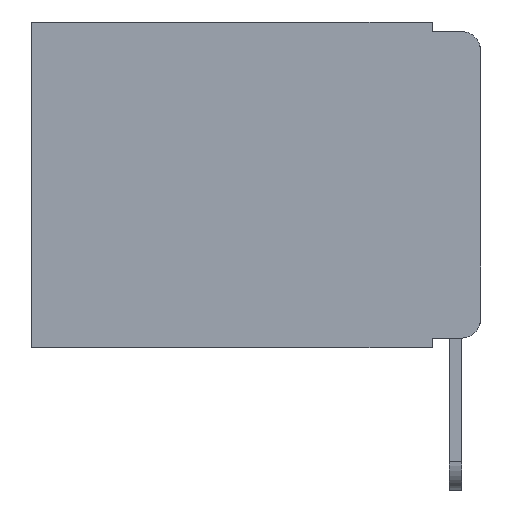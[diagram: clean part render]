
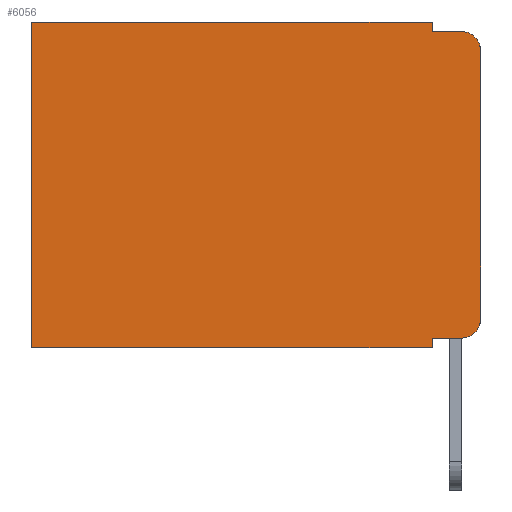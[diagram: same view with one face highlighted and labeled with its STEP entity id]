
A CAD part, left-side view. The second image highlights one B-rep face of the part: STEP entity #6056.
In plain terms, the highlighted planar face has unit normal (-1, 0, 0).
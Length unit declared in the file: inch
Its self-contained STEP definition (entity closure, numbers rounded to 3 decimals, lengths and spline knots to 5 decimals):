
#181 = CARTESIAN_POINT ( 'NONE',  ( 0.298, 0.051, -0.333 ) ) ;
#778 = PLANE ( 'NONE',  #12968 ) ;
#1369 = EDGE_CURVE ( 'NONE', #5572, #11298, #10958, .T. ) ;
#1847 = VECTOR ( 'NONE', #14663, 39.37008 ) ;
#2580 = CARTESIAN_POINT ( 'NONE',  ( 0.298, 0.02, -0.03 ) ) ;
#3357 = LINE ( 'NONE', #17226, #19488 ) ;
#3425 = DIRECTION ( 'NONE',  ( 0., 0., -1. ) ) ;
#3515 = CARTESIAN_POINT ( 'NONE',  ( 0.298, 0., -0.343 ) ) ;
#3864 = CARTESIAN_POINT ( 'NONE',  ( 0.298, 0.473, 0. ) ) ;
#4097 = EDGE_CURVE ( 'NONE', #12033, #11298, #12627, .T. ) ;
#4200 = DIRECTION ( 'NONE',  ( 0., 0., -1. ) ) ;
#4213 = EDGE_CURVE ( 'NONE', #16299, #5541, #19258, .T. ) ;
#4324 = VECTOR ( 'NONE', #3425, 39.37008 ) ;
#4493 = EDGE_CURVE ( 'NONE', #6920, #5959, #15123, .T. ) ;
#4494 = ORIENTED_EDGE ( 'NONE', *, *, #1369, .F. ) ;
#4986 = VERTEX_POINT ( 'NONE', #16802 ) ;
#5541 = VERTEX_POINT ( 'NONE', #6216 ) ;
#5571 = VECTOR ( 'NONE', #18722, 39.37008 ) ;
#5572 = VERTEX_POINT ( 'NONE', #7860 ) ;
#5959 = VERTEX_POINT ( 'NONE', #6481 ) ;
#6010 = EDGE_CURVE ( 'NONE', #5959, #4986, #3357, .T. ) ;
#6024 = ORIENTED_EDGE ( 'NONE', *, *, #19895, .T. ) ;
#6056 = ADVANCED_FACE ( 'NONE', ( #15126 ), #778, .F. ) ;
#6216 = CARTESIAN_POINT ( 'NONE',  ( 0.298, 0., -0.313 ) ) ;
#6302 = EDGE_CURVE ( 'NONE', #15396, #5572, #16956, .T. ) ;
#6419 = CARTESIAN_POINT ( 'NONE',  ( 0.298, 0.473, 0. ) ) ;
#6420 = VECTOR ( 'NONE', #18588, 39.37008 ) ;
#6481 = CARTESIAN_POINT ( 'NONE',  ( 0.298, 0.051, -0.01 ) ) ;
#6900 = CARTESIAN_POINT ( 'NONE',  ( 0.298, 0., -0.03 ) ) ;
#6920 = VERTEX_POINT ( 'NONE', #14558 ) ;
#7513 = ORIENTED_EDGE ( 'NONE', *, *, #9626, .T. ) ;
#7668 = CARTESIAN_POINT ( 'NONE',  ( 0.298, 0.051, 0. ) ) ;
#7860 = CARTESIAN_POINT ( 'NONE',  ( 0.298, 0.051, -0.343 ) ) ;
#8318 = CARTESIAN_POINT ( 'NONE',  ( 0.298, 0., 0. ) ) ;
#8385 = VECTOR ( 'NONE', #18546, 39.37008 ) ;
#8697 = CARTESIAN_POINT ( 'NONE',  ( 0.298, 0.02, -0.313 ) ) ;
#9000 = ORIENTED_EDGE ( 'NONE', *, *, #6010, .F. ) ;
#9464 = LINE ( 'NONE', #181, #13202 ) ;
#9626 = EDGE_CURVE ( 'NONE', #16299, #4986, #10755, .T. ) ;
#9820 = LINE ( 'NONE', #17260, #5571 ) ;
#10168 = DIRECTION ( 'NONE',  ( 0., 0., -1. ) ) ;
#10313 = DIRECTION ( 'NONE',  ( 0., 0., -1. ) ) ;
#10755 = CIRCLE ( 'NONE', #10894, 0.02 ) ;
#10881 = VECTOR ( 'NONE', #17714, 39.37008 ) ;
#10894 = AXIS2_PLACEMENT_3D ( 'NONE', #2580, #13806, #4200 ) ;
#10958 = LINE ( 'NONE', #3515, #1847 ) ;
#11298 = VERTEX_POINT ( 'NONE', #19575 ) ;
#11922 = CARTESIAN_POINT ( 'NONE',  ( 0.298, 0.051, -0.333 ) ) ;
#12033 = VERTEX_POINT ( 'NONE', #6419 ) ;
#12627 = LINE ( 'NONE', #3864, #8385 ) ;
#12968 = AXIS2_PLACEMENT_3D ( 'NONE', #16601, #16512, #10168 ) ;
#13007 = ORIENTED_EDGE ( 'NONE', *, *, #4493, .F. ) ;
#13202 = VECTOR ( 'NONE', #17743, 39.37008 ) ;
#13381 = CIRCLE ( 'NONE', #17999, 0.02 ) ;
#13806 = DIRECTION ( 'NONE',  ( -1., 0., 0. ) ) ;
#14118 = DIRECTION ( 'NONE',  ( 0., -1., 0. ) ) ;
#14284 = ORIENTED_EDGE ( 'NONE', *, *, #14832, .T. ) ;
#14518 = ORIENTED_EDGE ( 'NONE', *, *, #6302, .F. ) ;
#14558 = CARTESIAN_POINT ( 'NONE',  ( 0.298, 0.051, 0. ) ) ;
#14663 = DIRECTION ( 'NONE',  ( 0., 1., 0. ) ) ;
#14832 = EDGE_CURVE ( 'NONE', #15396, #15092, #9464, .T. ) ;
#15092 = VERTEX_POINT ( 'NONE', #15667 ) ;
#15123 = LINE ( 'NONE', #7668, #10881 ) ;
#15126 = FACE_OUTER_BOUND ( 'NONE', #19796, .T. ) ;
#15396 = VERTEX_POINT ( 'NONE', #11922 ) ;
#15667 = CARTESIAN_POINT ( 'NONE',  ( 0.298, 0.02, -0.333 ) ) ;
#15732 = ORIENTED_EDGE ( 'NONE', *, *, #18782, .T. ) ;
#16299 = VERTEX_POINT ( 'NONE', #6900 ) ;
#16403 = ORIENTED_EDGE ( 'NONE', *, *, #4097, .T. ) ;
#16512 = DIRECTION ( 'NONE',  ( 1., 0., 0. ) ) ;
#16601 = CARTESIAN_POINT ( 'NONE',  ( 0.298, 0., 0. ) ) ;
#16802 = CARTESIAN_POINT ( 'NONE',  ( 0.298, 0.02, -0.01 ) ) ;
#16956 = LINE ( 'NONE', #17228, #4324 ) ;
#17226 = CARTESIAN_POINT ( 'NONE',  ( 0.298, 0.051, -0.01 ) ) ;
#17228 = CARTESIAN_POINT ( 'NONE',  ( 0.298, 0.051, 0. ) ) ;
#17260 = CARTESIAN_POINT ( 'NONE',  ( 0.298, 0., 0. ) ) ;
#17714 = DIRECTION ( 'NONE',  ( 0., 0., -1. ) ) ;
#17743 = DIRECTION ( 'NONE',  ( 0., -1., 0. ) ) ;
#17999 = AXIS2_PLACEMENT_3D ( 'NONE', #8697, #19487, #10313 ) ;
#18546 = DIRECTION ( 'NONE',  ( 0., 0., -1. ) ) ;
#18588 = DIRECTION ( 'NONE',  ( 0., 0., -1. ) ) ;
#18722 = DIRECTION ( 'NONE',  ( 0., 1., 0. ) ) ;
#18782 = EDGE_CURVE ( 'NONE', #15092, #5541, #13381, .T. ) ;
#19258 = LINE ( 'NONE', #8318, #6420 ) ;
#19487 = DIRECTION ( 'NONE',  ( -1., 0., 0. ) ) ;
#19488 = VECTOR ( 'NONE', #14118, 39.37008 ) ;
#19575 = CARTESIAN_POINT ( 'NONE',  ( 0.298, 0.473, -0.343 ) ) ;
#19796 = EDGE_LOOP ( 'NONE', ( #20541, #7513, #9000, #13007, #6024, #16403, #4494, #14518, #14284, #15732 ) ) ;
#19895 = EDGE_CURVE ( 'NONE', #6920, #12033, #9820, .T. ) ;
#20541 = ORIENTED_EDGE ( 'NONE', *, *, #4213, .F. ) ;
